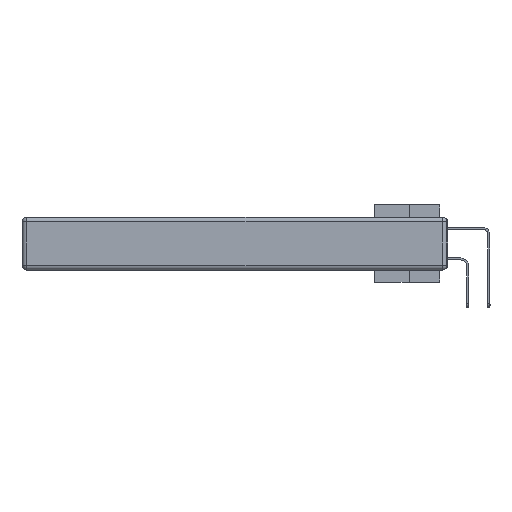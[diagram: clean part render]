
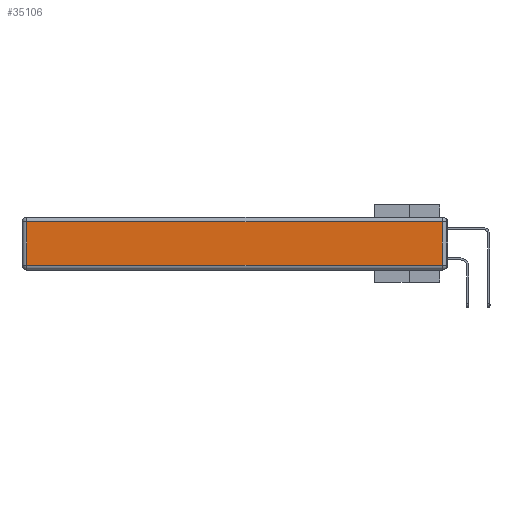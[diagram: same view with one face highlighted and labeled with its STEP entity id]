
A CAD part, left-side view. The second image highlights one B-rep face of the part: STEP entity #35106.
In plain terms, the highlighted planar face has unit normal (-1, 0, 0).
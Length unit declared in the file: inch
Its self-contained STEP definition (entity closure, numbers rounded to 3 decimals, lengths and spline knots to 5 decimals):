
#554 = CARTESIAN_POINT ( 'NONE',  ( 0., 0.03, -0.03 ) ) ;
#1511 = VECTOR ( 'NONE', #2810, 39.37008 ) ;
#1583 = CARTESIAN_POINT ( 'NONE',  ( 0., 0., -0.343 ) ) ;
#1745 = EDGE_CURVE ( 'NONE', #28573, #15148, #37342, .T. ) ;
#2487 = VERTEX_POINT ( 'NONE', #554 ) ;
#2810 = DIRECTION ( 'NONE',  ( 0., 0., 1. ) ) ;
#3706 = EDGE_LOOP ( 'NONE', ( #39625, #18339, #25390, #30635 ) ) ;
#5256 = LINE ( 'NONE', #39654, #30406 ) ;
#6617 = EDGE_CURVE ( 'NONE', #2487, #28573, #5256, .T. ) ;
#6918 = DIRECTION ( 'NONE',  ( 0., 0., -1. ) ) ;
#8867 = DIRECTION ( 'NONE',  ( 0., 1., 0. ) ) ;
#9911 = CARTESIAN_POINT ( 'NONE',  ( 0., 2.72, -0.03 ) ) ;
#12607 = AXIS2_PLACEMENT_3D ( 'NONE', #1583, #35665, #23205 ) ;
#15148 = VERTEX_POINT ( 'NONE', #22895 ) ;
#16425 = CARTESIAN_POINT ( 'NONE',  ( 0., 0., -0.313 ) ) ;
#16649 = LINE ( 'NONE', #16425, #30236 ) ;
#16811 = PLANE ( 'NONE',  #12607 ) ;
#17976 = VECTOR ( 'NONE', #6918, 39.37008 ) ;
#18339 = ORIENTED_EDGE ( 'NONE', *, *, #35340, .T. ) ;
#20132 = EDGE_CURVE ( 'NONE', #15148, #37730, #16649, .T. ) ;
#22895 = CARTESIAN_POINT ( 'NONE',  ( 0., 2.72, -0.313 ) ) ;
#23205 = DIRECTION ( 'NONE',  ( 0., 0., 1. ) ) ;
#25390 = ORIENTED_EDGE ( 'NONE', *, *, #6617, .T. ) ;
#28573 = VERTEX_POINT ( 'NONE', #9911 ) ;
#30236 = VECTOR ( 'NONE', #38097, 39.37008 ) ;
#30406 = VECTOR ( 'NONE', #8867, 39.37008 ) ;
#30635 = ORIENTED_EDGE ( 'NONE', *, *, #1745, .T. ) ;
#33484 = CARTESIAN_POINT ( 'NONE',  ( 0., 0.03, -0.343 ) ) ;
#33896 = FACE_OUTER_BOUND ( 'NONE', #3706, .T. ) ;
#35035 = CARTESIAN_POINT ( 'NONE',  ( 0., 2.72, -0.343 ) ) ;
#35106 = ADVANCED_FACE ( 'NONE', ( #33896 ), #16811, .T. ) ;
#35340 = EDGE_CURVE ( 'NONE', #37730, #2487, #38742, .T. ) ;
#35665 = DIRECTION ( 'NONE',  ( -1., 0., 0. ) ) ;
#36473 = CARTESIAN_POINT ( 'NONE',  ( 0., 0.03, -0.313 ) ) ;
#37342 = LINE ( 'NONE', #35035, #17976 ) ;
#37730 = VERTEX_POINT ( 'NONE', #36473 ) ;
#38097 = DIRECTION ( 'NONE',  ( 0., -1., 0. ) ) ;
#38742 = LINE ( 'NONE', #33484, #1511 ) ;
#39625 = ORIENTED_EDGE ( 'NONE', *, *, #20132, .T. ) ;
#39654 = CARTESIAN_POINT ( 'NONE',  ( 0., 2.75, -0.03 ) ) ;
